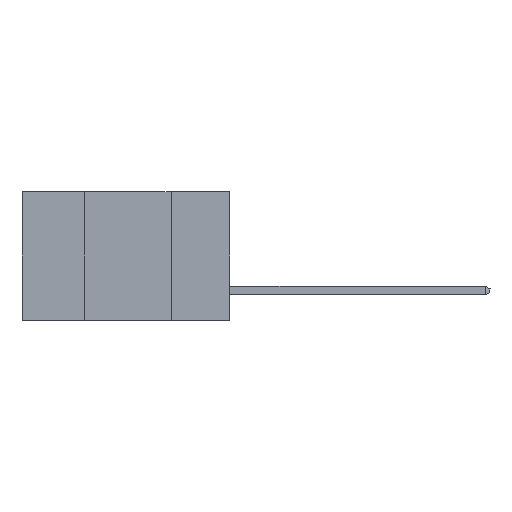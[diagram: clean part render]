
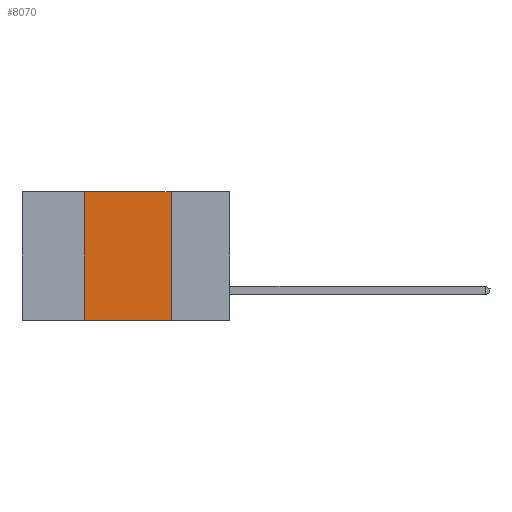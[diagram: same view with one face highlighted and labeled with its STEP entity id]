
A CAD part, left-side view. The second image highlights one B-rep face of the part: STEP entity #8070.
In plain terms, the highlighted planar face has unit normal (-1, 0, 0).
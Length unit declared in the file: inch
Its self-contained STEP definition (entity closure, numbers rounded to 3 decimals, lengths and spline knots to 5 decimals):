
#125 = DIRECTION ( 'NONE',  ( 0., 0., -1. ) ) ;
#260 = DIRECTION ( 'NONE',  ( 0., -1., 0. ) ) ;
#299 = CARTESIAN_POINT ( 'NONE',  ( 0., 0.6, 0. ) ) ;
#507 = VECTOR ( 'NONE', #10146, 39.37008 ) ;
#1089 = PLANE ( 'NONE',  #6952 ) ;
#2827 = VECTOR ( 'NONE', #7213, 39.37008 ) ;
#3857 = CARTESIAN_POINT ( 'NONE',  ( 0., 0.6, 0. ) ) ;
#4583 = DIRECTION ( 'NONE',  ( 1., 0., 0. ) ) ;
#5084 = EDGE_CURVE ( 'NONE', #9805, #8766, #7488, .T. ) ;
#5211 = VECTOR ( 'NONE', #260, 39.37008 ) ;
#5521 = LINE ( 'NONE', #3857, #5211 ) ;
#5706 = ORIENTED_EDGE ( 'NONE', *, *, #8474, .T. ) ;
#6736 = ORIENTED_EDGE ( 'NONE', *, *, #8148, .F. ) ;
#6952 = AXIS2_PLACEMENT_3D ( 'NONE', #299, #4583, #125 ) ;
#7001 = CARTESIAN_POINT ( 'NONE',  ( 0., 0.17, -0.37 ) ) ;
#7059 = LINE ( 'NONE', #7001, #2827 ) ;
#7097 = LINE ( 'NONE', #8734, #8457 ) ;
#7213 = DIRECTION ( 'NONE',  ( 0., 0., -1. ) ) ;
#7429 = EDGE_LOOP ( 'NONE', ( #6736, #10523, #10537, #5706 ) ) ;
#7488 = LINE ( 'NONE', #8498, #507 ) ;
#7989 = DIRECTION ( 'NONE',  ( 0., -1., 0. ) ) ;
#8070 = ADVANCED_FACE ( 'NONE', ( #10560 ), #1089, .F. ) ;
#8148 = EDGE_CURVE ( 'NONE', #10843, #9333, #7059, .T. ) ;
#8457 = VECTOR ( 'NONE', #7989, 39.37008 ) ;
#8474 = EDGE_CURVE ( 'NONE', #9805, #9333, #7097, .T. ) ;
#8498 = CARTESIAN_POINT ( 'NONE',  ( 0., 0.42, -0.37 ) ) ;
#8734 = CARTESIAN_POINT ( 'NONE',  ( 0., 0.6, -0.37 ) ) ;
#8766 = VERTEX_POINT ( 'NONE', #10408 ) ;
#8938 = EDGE_CURVE ( 'NONE', #8766, #10843, #5521, .T. ) ;
#9333 = VERTEX_POINT ( 'NONE', #9375 ) ;
#9375 = CARTESIAN_POINT ( 'NONE',  ( 0., 0.17, -0.37 ) ) ;
#9805 = VERTEX_POINT ( 'NONE', #10220 ) ;
#10146 = DIRECTION ( 'NONE',  ( 0., 0., 1. ) ) ;
#10220 = CARTESIAN_POINT ( 'NONE',  ( 0., 0.42, -0.37 ) ) ;
#10408 = CARTESIAN_POINT ( 'NONE',  ( 0., 0.42, 0. ) ) ;
#10523 = ORIENTED_EDGE ( 'NONE', *, *, #8938, .F. ) ;
#10537 = ORIENTED_EDGE ( 'NONE', *, *, #5084, .F. ) ;
#10560 = FACE_OUTER_BOUND ( 'NONE', #7429, .T. ) ;
#10830 = CARTESIAN_POINT ( 'NONE',  ( 0., 0.17, 0. ) ) ;
#10843 = VERTEX_POINT ( 'NONE', #10830 ) ;
